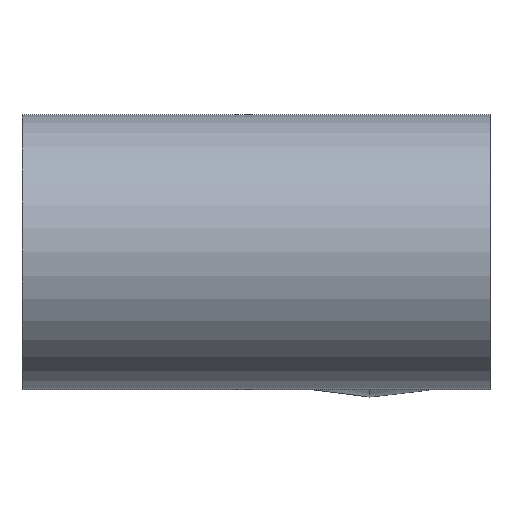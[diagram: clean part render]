
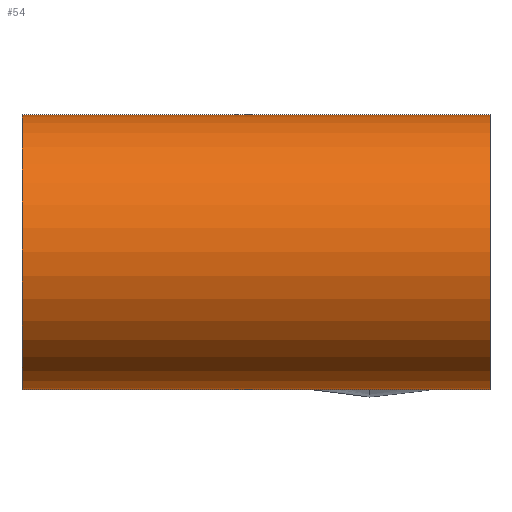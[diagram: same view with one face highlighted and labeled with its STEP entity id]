
A CAD part, top view. The second image highlights one B-rep face of the part: STEP entity #54.
In plain terms, the highlighted cylindrical face has radius 11.45 mm (diameter 22.9 mm), a partial arc.
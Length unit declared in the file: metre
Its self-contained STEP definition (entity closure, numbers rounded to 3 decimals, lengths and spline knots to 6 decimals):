
#54=ADVANCED_FACE('0:59',(#136),#137,.T.);
#136=FACE_OUTER_BOUND('',#344,.T.);
#137=CYLINDRICAL_SURFACE('',#345,0.01145);
#344=EDGE_LOOP('',(#4489,#4490,#4491,#4492));
#345=AXIS2_PLACEMENT_3D('',#4493,#4494,#4495);
#4489=ORIENTED_EDGE('',*,*,#5014,.F.);
#4490=ORIENTED_EDGE('',*,*,#5015,.T.);
#4491=ORIENTED_EDGE('',*,*,#5016,.F.);
#4492=ORIENTED_EDGE('',*,*,#5017,.F.);
#4493=CARTESIAN_POINT('',(0.101318,0.0472,0.0));
#4494=DIRECTION('',(1.0,0.0,0.0));
#4495=DIRECTION('',(0.0,1.0,0.0));
#5014=EDGE_CURVE('',#5225,#5226,#5227,.T.);
#5015=EDGE_CURVE('0:555',#5225,#5228,#5229,.T.);
#5016=EDGE_CURVE('',#5230,#5228,#5231,.T.);
#5017=EDGE_CURVE('0:546',#5226,#5230,#5232,.T.);
#5225=VERTEX_POINT('',#5726);
#5226=VERTEX_POINT('',#5727);
#5227=LINE('',#5728,#5729);
#5228=VERTEX_POINT('',#5730);
#5229=CIRCLE('',#5731,0.01145);
#5230=VERTEX_POINT('',#5732);
#5231=LINE('',#5733,#5734);
#5232=CIRCLE('',#5735,0.01145);
#5726=CARTESIAN_POINT('',(0.062318,0.05865,0.0));
#5727=CARTESIAN_POINT('',(0.101318,0.05865,0.));
#5728=CARTESIAN_POINT('',(0.101318,0.05865,0.));
#5729=VECTOR('',#6912,1.0);
#5730=CARTESIAN_POINT('',(0.062318,0.03575,0.));
#5731=AXIS2_PLACEMENT_3D('',#6913,#6914,#6915);
#5732=CARTESIAN_POINT('',(0.101318,0.03575,0.));
#5733=CARTESIAN_POINT('',(0.101318,0.03575,0.));
#5734=VECTOR('',#6916,1.0);
#5735=AXIS2_PLACEMENT_3D('',#6917,#6918,#6919);
#6912=DIRECTION('',(1.0,0.0,0.0));
#6913=CARTESIAN_POINT('',(0.062318,0.0472,0.0));
#6914=DIRECTION('',(1.0,0.0,0.0));
#6915=DIRECTION('',(0.0,1.0,0.0));
#6916=DIRECTION('',(-1.0,-0.0,-0.0));
#6917=CARTESIAN_POINT('',(0.101318,0.0472,0.0));
#6918=DIRECTION('',(1.0,0.0,0.0));
#6919=DIRECTION('',(0.0,1.0,0.0));
